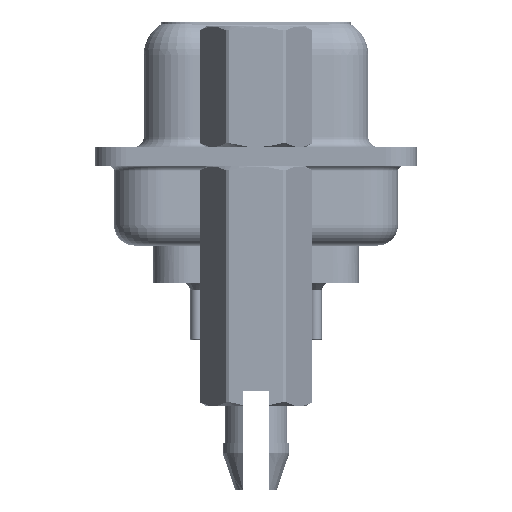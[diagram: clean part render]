
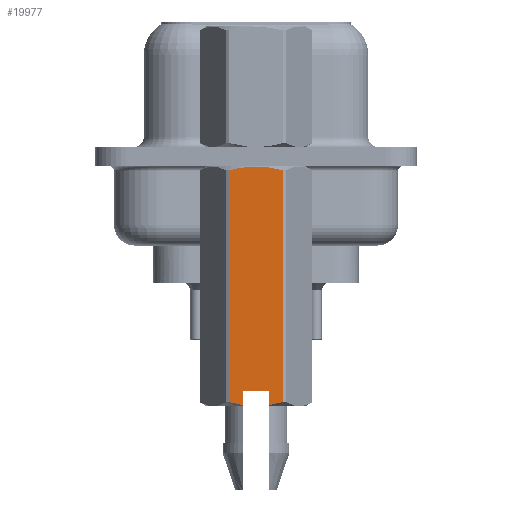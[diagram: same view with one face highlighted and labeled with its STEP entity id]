
A CAD part, left-side view. The second image highlights one B-rep face of the part: STEP entity #19977.
In plain terms, the highlighted planar face has unit normal (-1, 0, 0).
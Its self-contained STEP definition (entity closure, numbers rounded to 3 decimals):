
#22 = ORIENTED_EDGE ( 'NONE', *, *, #48263, .T. ) ;
#393 = ORIENTED_EDGE ( 'NONE', *, *, #40238, .T. ) ;
#909 = CARTESIAN_POINT ( 'NONE',  ( -2.381, -0.428, -0.485 ) ) ;
#1894 = CARTESIAN_POINT ( 'NONE',  ( -2.381, -0.625, -11.885 ) ) ;
#2430 = CARTESIAN_POINT ( 'NONE',  ( -2.381, -1.273, 0.581 ) ) ;
#3151 = LINE ( 'NONE', #2430, #48410 ) ;
#3269 = VERTEX_POINT ( 'NONE', #15345 ) ;
#4178 = ORIENTED_EDGE ( 'NONE', *, *, #44988, .F. ) ;
#4701 = CARTESIAN_POINT ( 'NONE',  ( -2.381, 0.432, -0.485 ) ) ;
#4714 = EDGE_LOOP ( 'NONE', ( #6432, #4178, #22, #30431, #16054, #43748, #393, #39604, #35707 ) ) ;
#4779 = CARTESIAN_POINT ( 'NONE',  ( -2.381, 0., -0.468 ) ) ;
#4962 = B_SPLINE_CURVE_WITH_KNOTS ( 'NONE', 3,
 ( #42605, #19848, #4701, #31266, #8558, #35105 ),
 .UNSPECIFIED., .F., .F.,
 ( 4, 2, 4 ),
 ( 0.004, 0.004, 0.005 ),
 .UNSPECIFIED. ) ;
#6432 = ORIENTED_EDGE ( 'NONE', *, *, #43293, .F. ) ;
#7180 = VECTOR ( 'NONE', #32933, 1000. ) ;
#7844 = B_SPLINE_CURVE_WITH_KNOTS ( 'NONE', 3,
 ( #19928, #42680, #23700, #909, #27498, #4779 ),
 .UNSPECIFIED., .F., .F.,
 ( 4, 2, 4 ),
 ( 0.003, 0.003, 0.004 ),
 .UNSPECIFIED. ) ;
#8141 = DIRECTION ( 'NONE',  ( 0., 0., -1. ) ) ;
#8558 = CARTESIAN_POINT ( 'NONE',  ( -2.381, 1.066, -0.596 ) ) ;
#9368 = VERTEX_POINT ( 'NONE', #32482 ) ;
#10926 = DIRECTION ( 'NONE',  ( 0., 0., -1. ) ) ;
#11101 = AXIS2_PLACEMENT_3D ( 'NONE', #31389, #16294, #42886 ) ;
#13019 = CARTESIAN_POINT ( 'NONE',  ( -2.381, 1.273, -0.652 ) ) ;
#14349 = CARTESIAN_POINT ( 'NONE',  ( -2.381, 0.845, -11.853 ) ) ;
#14687 = EDGE_CURVE ( 'NONE', #41203, #3269, #7844, .T. ) ;
#15345 = CARTESIAN_POINT ( 'NONE',  ( -2.381, 0., -0.468 ) ) ;
#16054 = ORIENTED_EDGE ( 'NONE', *, *, #44025, .T. ) ;
#16294 = DIRECTION ( 'NONE',  ( -1., 0., 0. ) ) ;
#16726 = EDGE_CURVE ( 'NONE', #34764, #22275, #34644, .T. ) ;
#17367 = CARTESIAN_POINT ( 'NONE',  ( -2.381, 1.273, -11.748 ) ) ;
#18487 = CARTESIAN_POINT ( 'NONE',  ( -2.381, 1.273, -11.748 ) ) ;
#19848 = CARTESIAN_POINT ( 'NONE',  ( -2.381, 0.215, -0.468 ) ) ;
#19928 = CARTESIAN_POINT ( 'NONE',  ( -2.381, -1.273, -0.652 ) ) ;
#19977 = ADVANCED_FACE ( 'NONE', ( #21207 ), #35063, .T. ) ;
#19981 = EDGE_CURVE ( 'NONE', #45857, #43939, #42238, .T. ) ;
#20124 = CARTESIAN_POINT ( 'NONE',  ( -2.381, -1.06, -11.806 ) ) ;
#21027 = LINE ( 'NONE', #44450, #7180 ) ;
#21207 = FACE_OUTER_BOUND ( 'NONE', #4714, .T. ) ;
#22275 = VERTEX_POINT ( 'NONE', #31131 ) ;
#22492 = CARTESIAN_POINT ( 'NONE',  ( -2.381, -1.273, -0.652 ) ) ;
#23700 = CARTESIAN_POINT ( 'NONE',  ( -2.381, -0.853, -0.549 ) ) ;
#23914 = CARTESIAN_POINT ( 'NONE',  ( -2.381, -0.625, -11.885 ) ) ;
#24062 = VERTEX_POINT ( 'NONE', #13019 ) ;
#25219 = VECTOR ( 'NONE', #8141, 1000. ) ;
#25220 = DIRECTION ( 'NONE',  ( 0., 0., 1. ) ) ;
#27498 = CARTESIAN_POINT ( 'NONE',  ( -2.381, -0.215, -0.468 ) ) ;
#28238 = DIRECTION ( 'NONE',  ( 0., 0., -1. ) ) ;
#28357 = CARTESIAN_POINT ( 'NONE',  ( -2.381, -1.273, -11.748 ) ) ;
#28498 = CARTESIAN_POINT ( 'NONE',  ( -2.381, -1.273, -11.748 ) ) ;
#29698 = EDGE_CURVE ( 'NONE', #24062, #34764, #45506, .T. ) ;
#30431 = ORIENTED_EDGE ( 'NONE', *, *, #19981, .T. ) ;
#31131 = CARTESIAN_POINT ( 'NONE',  ( -2.381, 0.625, -11.885 ) ) ;
#31266 = CARTESIAN_POINT ( 'NONE',  ( -2.381, 0.858, -0.55 ) ) ;
#31389 = CARTESIAN_POINT ( 'NONE',  ( -2.381, -1.375, -0.45 ) ) ;
#31959 = CARTESIAN_POINT ( 'NONE',  ( -2.381, 0.625, -11.2 ) ) ;
#32349 = LINE ( 'NONE', #31959, #42472 ) ;
#32482 = CARTESIAN_POINT ( 'NONE',  ( -2.381, -0.625, -11.2 ) ) ;
#32933 = DIRECTION ( 'NONE',  ( 0., 1., 0. ) ) ;
#33644 = CARTESIAN_POINT ( 'NONE',  ( -2.381, -0.625, -11.2 ) ) ;
#33663 = LINE ( 'NONE', #33644, #34858 ) ;
#34644 = B_SPLINE_CURVE_WITH_KNOTS ( 'NONE', 3,
 ( #18487, #37415, #14349, #45084 ),
 .UNSPECIFIED., .F., .F.,
 ( 4, 4 ),
 ( 0.001, 0.002 ),
 .UNSPECIFIED. ) ;
#34764 = VERTEX_POINT ( 'NONE', #17367 ) ;
#34858 = VECTOR ( 'NONE', #10926, 1000. ) ;
#35063 = PLANE ( 'NONE',  #11101 ) ;
#35105 = CARTESIAN_POINT ( 'NONE',  ( -2.381, 1.273, -0.652 ) ) ;
#35707 = ORIENTED_EDGE ( 'NONE', *, *, #16726, .T. ) ;
#37415 = CARTESIAN_POINT ( 'NONE',  ( -2.381, 1.06, -11.806 ) ) ;
#38348 = VERTEX_POINT ( 'NONE', #45104 ) ;
#39604 = ORIENTED_EDGE ( 'NONE', *, *, #29698, .T. ) ;
#40238 = EDGE_CURVE ( 'NONE', #3269, #24062, #4962, .T. ) ;
#41203 = VERTEX_POINT ( 'NONE', #22492 ) ;
#42238 = B_SPLINE_CURVE_WITH_KNOTS ( 'NONE', 3,
 ( #23914, #46696, #20124, #28357 ),
 .UNSPECIFIED., .F., .F.,
 ( 4, 4 ),
 ( 0.003, 0.004 ),
 .UNSPECIFIED. ) ;
#42472 = VECTOR ( 'NONE', #28238, 1000. ) ;
#42605 = CARTESIAN_POINT ( 'NONE',  ( -2.381, 0., -0.468 ) ) ;
#42680 = CARTESIAN_POINT ( 'NONE',  ( -2.381, -1.065, -0.596 ) ) ;
#42886 = DIRECTION ( 'NONE',  ( 0., 0., 1. ) ) ;
#43293 = EDGE_CURVE ( 'NONE', #38348, #22275, #32349, .T. ) ;
#43748 = ORIENTED_EDGE ( 'NONE', *, *, #14687, .T. ) ;
#43939 = VERTEX_POINT ( 'NONE', #28498 ) ;
#44025 = EDGE_CURVE ( 'NONE', #43939, #41203, #3151, .T. ) ;
#44450 = CARTESIAN_POINT ( 'NONE',  ( -2.381, -0.625, -11.2 ) ) ;
#44988 = EDGE_CURVE ( 'NONE', #9368, #38348, #21027, .T. ) ;
#45084 = CARTESIAN_POINT ( 'NONE',  ( -2.381, 0.625, -11.885 ) ) ;
#45104 = CARTESIAN_POINT ( 'NONE',  ( -2.381, 0.625, -11.2 ) ) ;
#45506 = LINE ( 'NONE', #46024, #25219 ) ;
#45857 = VERTEX_POINT ( 'NONE', #1894 ) ;
#46024 = CARTESIAN_POINT ( 'NONE',  ( -2.381, 1.273, 0.581 ) ) ;
#46696 = CARTESIAN_POINT ( 'NONE',  ( -2.381, -0.842, -11.854 ) ) ;
#48263 = EDGE_CURVE ( 'NONE', #9368, #45857, #33663, .T. ) ;
#48410 = VECTOR ( 'NONE', #25220, 1000. ) ;
